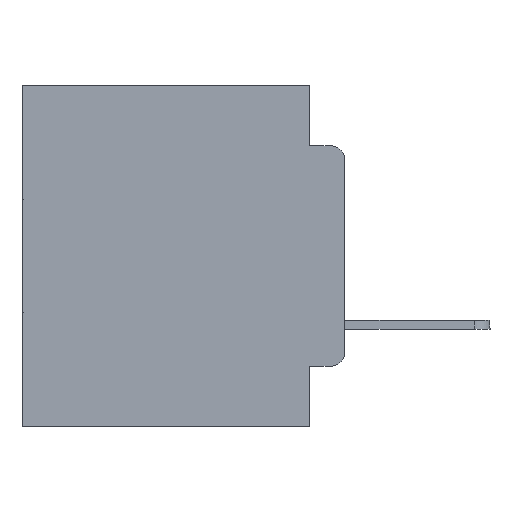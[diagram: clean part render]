
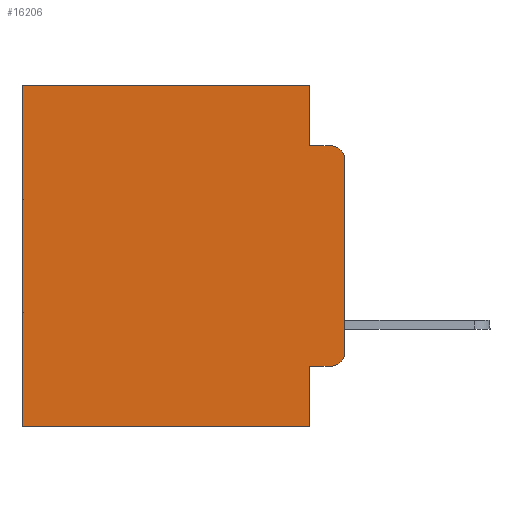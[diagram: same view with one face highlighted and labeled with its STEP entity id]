
A CAD part, left-side view. The second image highlights one B-rep face of the part: STEP entity #16206.
In plain terms, the highlighted planar face has unit normal (-1, 0, 0).
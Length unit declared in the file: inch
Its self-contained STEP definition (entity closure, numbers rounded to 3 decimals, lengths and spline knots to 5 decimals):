
#12 = VECTOR ( 'NONE', #20139, 39.37008 ) ;
#207 = CARTESIAN_POINT ( 'NONE',  ( 0.298, 0.473, 0. ) ) ;
#225 = LINE ( 'NONE', #2063, #546 ) ;
#322 = VERTEX_POINT ( 'NONE', #17441 ) ;
#345 = CARTESIAN_POINT ( 'NONE',  ( 0.298, 0.051, -0.5 ) ) ;
#546 = VECTOR ( 'NONE', #14095, 39.37008 ) ;
#1663 = DIRECTION ( 'NONE',  ( 0., 1., 0. ) ) ;
#1743 = ORIENTED_EDGE ( 'NONE', *, *, #9709, .T. ) ;
#2063 = CARTESIAN_POINT ( 'NONE',  ( 0.298, 0.051, -0.4115 ) ) ;
#2353 = CARTESIAN_POINT ( 'NONE',  ( 0.298, 0., -0.3915 ) ) ;
#2437 = CIRCLE ( 'NONE', #27972, 0.02 ) ;
#2834 = LINE ( 'NONE', #14868, #16668 ) ;
#3294 = LINE ( 'NONE', #207, #22457 ) ;
#3330 = EDGE_CURVE ( 'NONE', #25143, #16526, #22335, .T. ) ;
#4050 = DIRECTION ( 'NONE',  ( -1., 0., 0. ) ) ;
#4466 = LINE ( 'NONE', #21159, #11508 ) ;
#5205 = DIRECTION ( 'NONE',  ( 1., 0., 0. ) ) ;
#5282 = ORIENTED_EDGE ( 'NONE', *, *, #3330, .F. ) ;
#5546 = EDGE_CURVE ( 'NONE', #322, #25143, #2834, .T. ) ;
#5798 = DIRECTION ( 'NONE',  ( 0., 0., -1. ) ) ;
#6847 = VERTEX_POINT ( 'NONE', #23653 ) ;
#7825 = EDGE_CURVE ( 'NONE', #11497, #9926, #12682, .T. ) ;
#9176 = DIRECTION ( 'NONE',  ( -1., 0., 0. ) ) ;
#9709 = EDGE_CURVE ( 'NONE', #6847, #9850, #2437, .T. ) ;
#9850 = VERTEX_POINT ( 'NONE', #2353 ) ;
#9926 = VERTEX_POINT ( 'NONE', #22198 ) ;
#10119 = ORIENTED_EDGE ( 'NONE', *, *, #5546, .F. ) ;
#10259 = ORIENTED_EDGE ( 'NONE', *, *, #16312, .T. ) ;
#10789 = ORIENTED_EDGE ( 'NONE', *, *, #21051, .T. ) ;
#11402 = VERTEX_POINT ( 'NONE', #19830 ) ;
#11497 = VERTEX_POINT ( 'NONE', #15875 ) ;
#11508 = VECTOR ( 'NONE', #14200, 39.37008 ) ;
#11561 = EDGE_CURVE ( 'NONE', #11497, #9850, #4466, .T. ) ;
#11811 = CARTESIAN_POINT ( 'NONE',  ( 0.298, 0.051, 0. ) ) ;
#12032 = EDGE_LOOP ( 'NONE', ( #29295, #22873, #20218, #20445, #10259, #10789, #5282, #10119, #20016, #1743 ) ) ;
#12682 = CIRCLE ( 'NONE', #19515, 0.02 ) ;
#12932 = VERTEX_POINT ( 'NONE', #26576 ) ;
#13327 = EDGE_CURVE ( 'NONE', #23497, #9926, #15587, .T. ) ;
#14095 = DIRECTION ( 'NONE',  ( 0., -1., 0. ) ) ;
#14200 = DIRECTION ( 'NONE',  ( 0., 0., -1. ) ) ;
#14498 = LINE ( 'NONE', #11811, #26045 ) ;
#14537 = VECTOR ( 'NONE', #22073, 39.37008 ) ;
#14868 = CARTESIAN_POINT ( 'NONE',  ( 0.298, 0.051, 0. ) ) ;
#15238 = CARTESIAN_POINT ( 'NONE',  ( 0.298, 0., -0.5 ) ) ;
#15471 = DIRECTION ( 'NONE',  ( 0., 0., -1. ) ) ;
#15587 = LINE ( 'NONE', #22550, #12 ) ;
#15875 = CARTESIAN_POINT ( 'NONE',  ( 0.298, 0., -0.1085 ) ) ;
#16206 = ADVANCED_FACE ( 'NONE', ( #26437 ), #16787, .F. ) ;
#16312 = EDGE_CURVE ( 'NONE', #12932, #11402, #17839, .T. ) ;
#16526 = VERTEX_POINT ( 'NONE', #28387 ) ;
#16668 = VECTOR ( 'NONE', #28480, 39.37008 ) ;
#16787 = PLANE ( 'NONE',  #26597 ) ;
#16927 = DIRECTION ( 'NONE',  ( 0., 0., -1. ) ) ;
#17441 = CARTESIAN_POINT ( 'NONE',  ( 0.298, 0.051, -0.4115 ) ) ;
#17443 = CARTESIAN_POINT ( 'NONE',  ( 0.298, 0.02, -0.3915 ) ) ;
#17839 = LINE ( 'NONE', #22218, #14537 ) ;
#19515 = AXIS2_PLACEMENT_3D ( 'NONE', #25905, #9176, #23213 ) ;
#19830 = CARTESIAN_POINT ( 'NONE',  ( 0.298, 0.473, 0. ) ) ;
#20016 = ORIENTED_EDGE ( 'NONE', *, *, #23266, .T. ) ;
#20139 = DIRECTION ( 'NONE',  ( 0., -1., 0. ) ) ;
#20218 = ORIENTED_EDGE ( 'NONE', *, *, #13327, .F. ) ;
#20445 = ORIENTED_EDGE ( 'NONE', *, *, #23808, .F. ) ;
#21051 = EDGE_CURVE ( 'NONE', #11402, #16526, #3294, .T. ) ;
#21159 = CARTESIAN_POINT ( 'NONE',  ( 0.298, 0., 0. ) ) ;
#21186 = DIRECTION ( 'NONE',  ( 0., 0., -1. ) ) ;
#21633 = VECTOR ( 'NONE', #1663, 39.37008 ) ;
#22073 = DIRECTION ( 'NONE',  ( 0., 1., 0. ) ) ;
#22198 = CARTESIAN_POINT ( 'NONE',  ( 0.298, 0.02, -0.0885 ) ) ;
#22218 = CARTESIAN_POINT ( 'NONE',  ( 0.298, 0., 0. ) ) ;
#22335 = LINE ( 'NONE', #15238, #21633 ) ;
#22457 = VECTOR ( 'NONE', #21186, 39.37008 ) ;
#22550 = CARTESIAN_POINT ( 'NONE',  ( 0.298, 0.051, -0.0885 ) ) ;
#22873 = ORIENTED_EDGE ( 'NONE', *, *, #7825, .T. ) ;
#23213 = DIRECTION ( 'NONE',  ( 0., 0., -1. ) ) ;
#23266 = EDGE_CURVE ( 'NONE', #322, #6847, #225, .T. ) ;
#23497 = VERTEX_POINT ( 'NONE', #29052 ) ;
#23653 = CARTESIAN_POINT ( 'NONE',  ( 0.298, 0.02, -0.4115 ) ) ;
#23808 = EDGE_CURVE ( 'NONE', #12932, #23497, #14498, .T. ) ;
#25143 = VERTEX_POINT ( 'NONE', #345 ) ;
#25905 = CARTESIAN_POINT ( 'NONE',  ( 0.298, 0.02, -0.1085 ) ) ;
#26045 = VECTOR ( 'NONE', #16927, 39.37008 ) ;
#26437 = FACE_OUTER_BOUND ( 'NONE', #12032, .T. ) ;
#26576 = CARTESIAN_POINT ( 'NONE',  ( 0.298, 0.051, 0. ) ) ;
#26597 = AXIS2_PLACEMENT_3D ( 'NONE', #28270, #5205, #5798 ) ;
#27972 = AXIS2_PLACEMENT_3D ( 'NONE', #17443, #4050, #15471 ) ;
#28270 = CARTESIAN_POINT ( 'NONE',  ( 0.298, 0., 0. ) ) ;
#28387 = CARTESIAN_POINT ( 'NONE',  ( 0.298, 0.473, -0.5 ) ) ;
#28480 = DIRECTION ( 'NONE',  ( 0., 0., -1. ) ) ;
#29052 = CARTESIAN_POINT ( 'NONE',  ( 0.298, 0.051, -0.0885 ) ) ;
#29295 = ORIENTED_EDGE ( 'NONE', *, *, #11561, .F. ) ;
